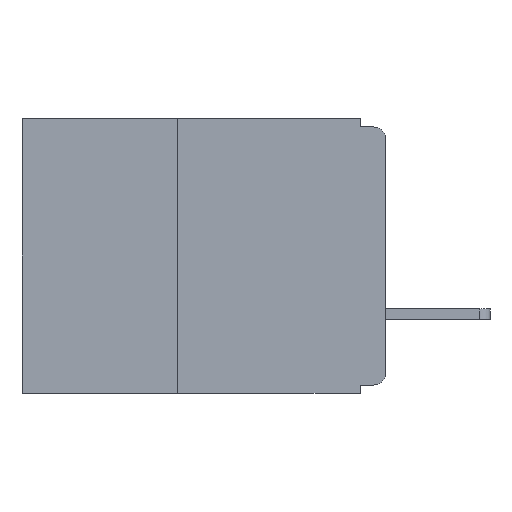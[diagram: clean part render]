
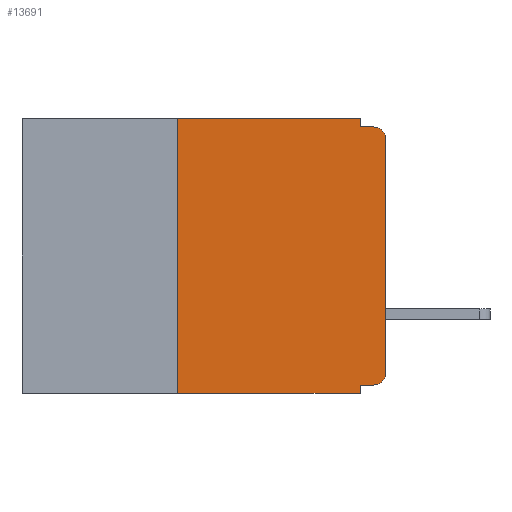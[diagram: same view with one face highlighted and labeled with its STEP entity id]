
A CAD part, left-side view. The second image highlights one B-rep face of the part: STEP entity #13691.
In plain terms, the highlighted planar face has unit normal (-1, 0, 0).
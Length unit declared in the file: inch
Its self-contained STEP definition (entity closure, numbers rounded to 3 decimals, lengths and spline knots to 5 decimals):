
#584 = CIRCLE ( 'NONE', #2812, 0.015 ) ;
#1240 = ORIENTED_EDGE ( 'NONE', *, *, #5165, .T. ) ;
#1513 = DIRECTION ( 'NONE',  ( 0., 0., -1. ) ) ;
#1516 = EDGE_CURVE ( 'NONE', #6236, #13336, #11206, .T. ) ;
#1754 = CARTESIAN_POINT ( 'NONE',  ( 0., 0.031, -0.33 ) ) ;
#1913 = ORIENTED_EDGE ( 'NONE', *, *, #3470, .F. ) ;
#2394 = DIRECTION ( 'NONE',  ( 0., 0., -1. ) ) ;
#2413 = EDGE_CURVE ( 'NONE', #11197, #4624, #14723, .T. ) ;
#2426 = DIRECTION ( 'NONE',  ( 0., -1., 0. ) ) ;
#2456 = VECTOR ( 'NONE', #2580, 39.37008 ) ;
#2551 = VERTEX_POINT ( 'NONE', #5219 ) ;
#2580 = DIRECTION ( 'NONE',  ( 0., -1., 0. ) ) ;
#2612 = CARTESIAN_POINT ( 'NONE',  ( 0., 0., -0.01 ) ) ;
#2682 = DIRECTION ( 'NONE',  ( 0., 0., 1. ) ) ;
#2802 = ORIENTED_EDGE ( 'NONE', *, *, #5798, .F. ) ;
#2812 = AXIS2_PLACEMENT_3D ( 'NONE', #8359, #8239, #8197 ) ;
#2890 = VERTEX_POINT ( 'NONE', #4586 ) ;
#3165 = LINE ( 'NONE', #6953, #10419 ) ;
#3399 = FACE_OUTER_BOUND ( 'NONE', #5899, .T. ) ;
#3470 = EDGE_CURVE ( 'NONE', #16274, #2551, #4132, .T. ) ;
#3482 = VECTOR ( 'NONE', #2682, 39.37008 ) ;
#3970 = AXIS2_PLACEMENT_3D ( 'NONE', #9695, #9764, #1513 ) ;
#3981 = VECTOR ( 'NONE', #2426, 39.37008 ) ;
#4132 = LINE ( 'NONE', #1754, #8579 ) ;
#4253 = ORIENTED_EDGE ( 'NONE', *, *, #14191, .F. ) ;
#4586 = CARTESIAN_POINT ( 'NONE',  ( 0., 0.031, -0.01 ) ) ;
#4624 = VERTEX_POINT ( 'NONE', #11850 ) ;
#4840 = VERTEX_POINT ( 'NONE', #16521 ) ;
#5165 = EDGE_CURVE ( 'NONE', #11849, #15839, #584, .T. ) ;
#5219 = CARTESIAN_POINT ( 'NONE',  ( 0., 0.031, -0.33 ) ) ;
#5798 = EDGE_CURVE ( 'NONE', #4840, #2890, #3165, .T. ) ;
#5899 = EDGE_LOOP ( 'NONE', ( #9199, #1240, #12778, #2802, #9877, #7520, #15946, #1913, #4253, #7825 ) ) ;
#6236 = VERTEX_POINT ( 'NONE', #15668 ) ;
#6263 = CARTESIAN_POINT ( 'NONE',  ( 0., 0., -0.305 ) ) ;
#6606 = VECTOR ( 'NONE', #12886, 39.37008 ) ;
#6861 = CARTESIAN_POINT ( 'NONE',  ( 0., 0.437, 0. ) ) ;
#6953 = CARTESIAN_POINT ( 'NONE',  ( 0., 0.031, 0. ) ) ;
#7017 = DIRECTION ( 'NONE',  ( 0., 0., -1. ) ) ;
#7121 = LINE ( 'NONE', #16188, #3482 ) ;
#7520 = ORIENTED_EDGE ( 'NONE', *, *, #2413, .F. ) ;
#7535 = EDGE_CURVE ( 'NONE', #2890, #15839, #16841, .T. ) ;
#7825 = ORIENTED_EDGE ( 'NONE', *, *, #1516, .T. ) ;
#7864 = LINE ( 'NONE', #10102, #6606 ) ;
#7933 = DIRECTION ( 'NONE',  ( 0., 0., -1. ) ) ;
#7956 = DIRECTION ( 'NONE',  ( -1., 0., 0. ) ) ;
#8197 = DIRECTION ( 'NONE',  ( 0., 0., -1. ) ) ;
#8239 = DIRECTION ( 'NONE',  ( -1., 0., 0. ) ) ;
#8359 = CARTESIAN_POINT ( 'NONE',  ( 0., 0.015, -0.025 ) ) ;
#8579 = VECTOR ( 'NONE', #2394, 39.37008 ) ;
#8823 = VECTOR ( 'NONE', #10090, 39.37008 ) ;
#9162 = CARTESIAN_POINT ( 'NONE',  ( 0., 0.015, -0.305 ) ) ;
#9180 = VECTOR ( 'NONE', #12230, 39.37008 ) ;
#9199 = ORIENTED_EDGE ( 'NONE', *, *, #9470, .T. ) ;
#9470 = EDGE_CURVE ( 'NONE', #13336, #11849, #7121, .T. ) ;
#9695 = CARTESIAN_POINT ( 'NONE',  ( 0., 0.437, 0. ) ) ;
#9764 = DIRECTION ( 'NONE',  ( 1., 0., 0. ) ) ;
#9877 = ORIENTED_EDGE ( 'NONE', *, *, #11165, .F. ) ;
#9932 = CARTESIAN_POINT ( 'NONE',  ( 0., 0.015, -0.01 ) ) ;
#10090 = DIRECTION ( 'NONE',  ( 0., 0., 1. ) ) ;
#10102 = CARTESIAN_POINT ( 'NONE',  ( 0., 0., -0.32 ) ) ;
#10419 = VECTOR ( 'NONE', #7017, 39.37008 ) ;
#10768 = LINE ( 'NONE', #14666, #3981 ) ;
#11165 = EDGE_CURVE ( 'NONE', #4624, #4840, #12739, .T. ) ;
#11197 = VERTEX_POINT ( 'NONE', #12165 ) ;
#11206 = CIRCLE ( 'NONE', #16276, 0.015 ) ;
#11849 = VERTEX_POINT ( 'NONE', #15086 ) ;
#11850 = CARTESIAN_POINT ( 'NONE',  ( 0., 0.25, 0. ) ) ;
#12165 = CARTESIAN_POINT ( 'NONE',  ( 0., 0.25, -0.33 ) ) ;
#12230 = DIRECTION ( 'NONE',  ( 0., -1., 0. ) ) ;
#12739 = LINE ( 'NONE', #6861, #9180 ) ;
#12778 = ORIENTED_EDGE ( 'NONE', *, *, #7535, .F. ) ;
#12886 = DIRECTION ( 'NONE',  ( 0., 1., 0. ) ) ;
#13336 = VERTEX_POINT ( 'NONE', #6263 ) ;
#13691 = ADVANCED_FACE ( 'NONE', ( #3399 ), #13734, .F. ) ;
#13734 = PLANE ( 'NONE',  #3970 ) ;
#13915 = CARTESIAN_POINT ( 'NONE',  ( 0., 0.25, -0.33 ) ) ;
#14191 = EDGE_CURVE ( 'NONE', #6236, #16274, #7864, .T. ) ;
#14666 = CARTESIAN_POINT ( 'NONE',  ( 0., 0.437, -0.33 ) ) ;
#14723 = LINE ( 'NONE', #13915, #8823 ) ;
#15086 = CARTESIAN_POINT ( 'NONE',  ( 0., 0., -0.025 ) ) ;
#15668 = CARTESIAN_POINT ( 'NONE',  ( 0., 0.015, -0.32 ) ) ;
#15839 = VERTEX_POINT ( 'NONE', #9932 ) ;
#15946 = ORIENTED_EDGE ( 'NONE', *, *, #16160, .T. ) ;
#16160 = EDGE_CURVE ( 'NONE', #11197, #2551, #10768, .T. ) ;
#16188 = CARTESIAN_POINT ( 'NONE',  ( 0., 0., 0. ) ) ;
#16274 = VERTEX_POINT ( 'NONE', #16296 ) ;
#16276 = AXIS2_PLACEMENT_3D ( 'NONE', #9162, #7956, #7933 ) ;
#16296 = CARTESIAN_POINT ( 'NONE',  ( 0., 0.031, -0.32 ) ) ;
#16521 = CARTESIAN_POINT ( 'NONE',  ( 0., 0.031, 0. ) ) ;
#16841 = LINE ( 'NONE', #2612, #2456 ) ;
